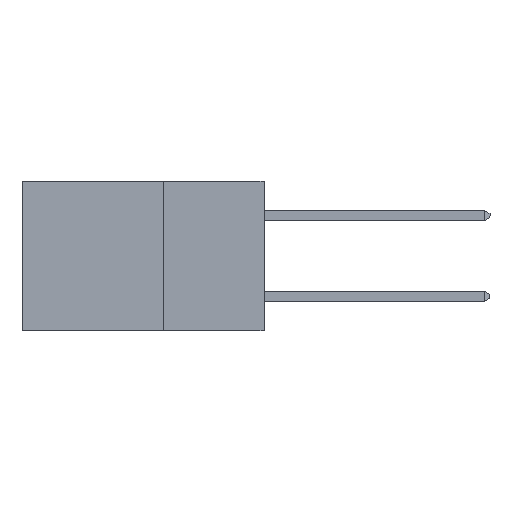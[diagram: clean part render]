
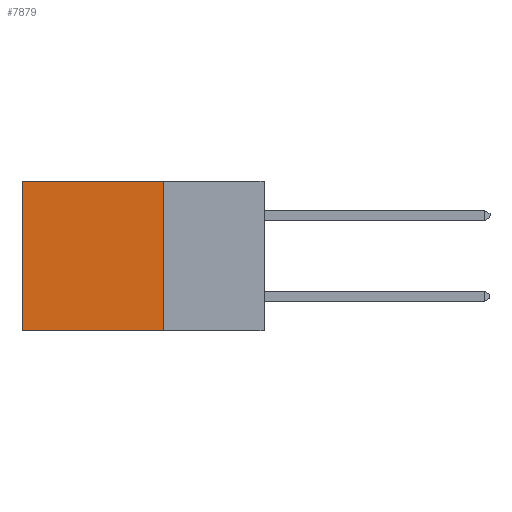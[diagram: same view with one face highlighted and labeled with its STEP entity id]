
A CAD part, left-side view. The second image highlights one B-rep face of the part: STEP entity #7879.
In plain terms, the highlighted planar face has unit normal (-1, 0, 0).
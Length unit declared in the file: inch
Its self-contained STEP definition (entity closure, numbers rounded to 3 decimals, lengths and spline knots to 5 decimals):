
#557 = EDGE_CURVE ( 'NONE', #1263, #28043, #24610, .T. ) ;
#1263 = VERTEX_POINT ( 'NONE', #20609 ) ;
#2890 = CARTESIAN_POINT ( 'NONE',  ( 0.298, 0.6, 0. ) ) ;
#3414 = ORIENTED_EDGE ( 'NONE', *, *, #557, .F. ) ;
#3619 = AXIS2_PLACEMENT_3D ( 'NONE', #20520, #5827, #23006 ) ;
#3790 = CARTESIAN_POINT ( 'NONE',  ( 0.298, 0.25, -0.37 ) ) ;
#4252 = EDGE_CURVE ( 'NONE', #1263, #28432, #23263, .T. ) ;
#5238 = DIRECTION ( 'NONE',  ( 0., 0., -1. ) ) ;
#5827 = DIRECTION ( 'NONE',  ( 1., 0., 0. ) ) ;
#6497 = CARTESIAN_POINT ( 'NONE',  ( 0.298, 0.25, -0.37 ) ) ;
#7762 = ORIENTED_EDGE ( 'NONE', *, *, #19654, .F. ) ;
#7879 = ADVANCED_FACE ( 'NONE', ( #22216 ), #13160, .F. ) ;
#8860 = DIRECTION ( 'NONE',  ( 0., 1., 0. ) ) ;
#8918 = ORIENTED_EDGE ( 'NONE', *, *, #29108, .T. ) ;
#10594 = DIRECTION ( 'NONE',  ( 0., 0., -1. ) ) ;
#11577 = VECTOR ( 'NONE', #10594, 39.37008 ) ;
#12207 = ORIENTED_EDGE ( 'NONE', *, *, #4252, .T. ) ;
#13160 = PLANE ( 'NONE',  #3619 ) ;
#15190 = VECTOR ( 'NONE', #8860, 39.37008 ) ;
#17851 = CARTESIAN_POINT ( 'NONE',  ( 0.298, 0.25, 0. ) ) ;
#18583 = CARTESIAN_POINT ( 'NONE',  ( 0.298, 0.25, 0. ) ) ;
#19654 = EDGE_CURVE ( 'NONE', #28043, #21793, #22638, .T. ) ;
#20520 = CARTESIAN_POINT ( 'NONE',  ( 0.298, 0.25, 0. ) ) ;
#20609 = CARTESIAN_POINT ( 'NONE',  ( 0.298, 0.25, 0. ) ) ;
#21695 = CARTESIAN_POINT ( 'NONE',  ( 0.298, 0.6, -0.37 ) ) ;
#21793 = VERTEX_POINT ( 'NONE', #21695 ) ;
#22216 = FACE_OUTER_BOUND ( 'NONE', #23311, .T. ) ;
#22638 = LINE ( 'NONE', #3790, #29945 ) ;
#23006 = DIRECTION ( 'NONE',  ( 0., 0., -1. ) ) ;
#23263 = LINE ( 'NONE', #18583, #15190 ) ;
#23311 = EDGE_LOOP ( 'NONE', ( #8918, #7762, #3414, #12207 ) ) ;
#24610 = LINE ( 'NONE', #17851, #11577 ) ;
#24907 = CARTESIAN_POINT ( 'NONE',  ( 0.298, 0.6, 0. ) ) ;
#24953 = LINE ( 'NONE', #24907, #31478 ) ;
#28043 = VERTEX_POINT ( 'NONE', #6497 ) ;
#28294 = DIRECTION ( 'NONE',  ( 0., 1., 0. ) ) ;
#28432 = VERTEX_POINT ( 'NONE', #2890 ) ;
#29108 = EDGE_CURVE ( 'NONE', #28432, #21793, #24953, .T. ) ;
#29945 = VECTOR ( 'NONE', #28294, 39.37008 ) ;
#31478 = VECTOR ( 'NONE', #5238, 39.37008 ) ;
